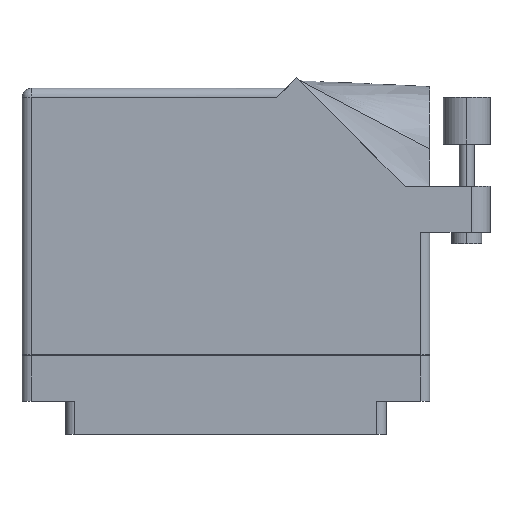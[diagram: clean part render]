
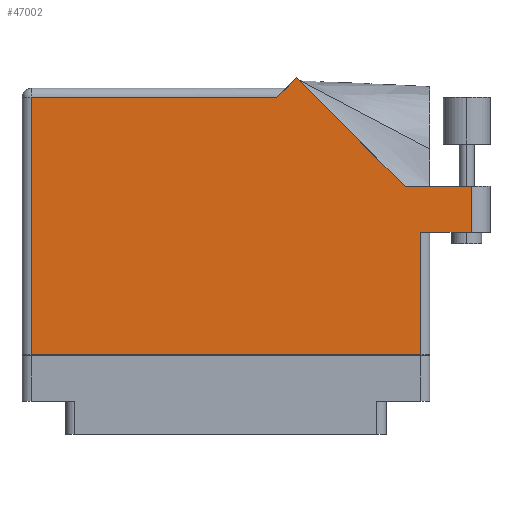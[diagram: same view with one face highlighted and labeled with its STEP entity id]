
A CAD part, front view. The second image highlights one B-rep face of the part: STEP entity #47002.
In plain terms, the highlighted face is planar.
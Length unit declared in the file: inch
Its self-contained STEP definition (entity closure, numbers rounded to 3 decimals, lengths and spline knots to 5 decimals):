
#1333 = VECTOR ( 'NONE', #36020, 39.37008 ) ;
#1382 = CARTESIAN_POINT ( 'NONE',  ( 1.297, 0.715, 0.617 ) ) ;
#3426 = DIRECTION ( 'NONE',  ( -0.707, -0.707, 0. ) ) ;
#3529 = DIRECTION ( 'NONE',  ( -0.707, 0.707, 0. ) ) ;
#4554 = CARTESIAN_POINT ( 'NONE',  ( -1.297, 1.613, 0.617 ) ) ;
#5613 = EDGE_CURVE ( 'NONE', #24596, #61906, #36556, .T. ) ;
#5716 = VECTOR ( 'NONE', #3529, 39.37008 ) ;
#6157 = LINE ( 'NONE', #23024, #23441 ) ;
#6387 = VERTEX_POINT ( 'NONE', #10628 ) ;
#7170 = DIRECTION ( 'NONE',  ( -1., 0., 0. ) ) ;
#8017 = VERTEX_POINT ( 'NONE', #4554 ) ;
#8140 = LINE ( 'NONE', #24655, #5716 ) ;
#8535 = VECTOR ( 'NONE', #12633, 39.37008 ) ;
#9769 = VECTOR ( 'NONE', #3426, 39.37008 ) ;
#10628 = CARTESIAN_POINT ( 'NONE',  ( 0.46971, 1.74571, 0.617 ) ) ;
#12124 = EDGE_CURVE ( 'NONE', #60755, #61768, #32189, .T. ) ;
#12433 = FACE_OUTER_BOUND ( 'NONE', #34349, .T. ) ;
#12633 = DIRECTION ( 'NONE',  ( 0., 1., 0. ) ) ;
#13409 = DIRECTION ( 'NONE',  ( 1., 0., 0. ) ) ;
#15849 = VECTOR ( 'NONE', #68060, 39.37008 ) ;
#16316 = ORIENTED_EDGE ( 'NONE', *, *, #49561, .T. ) ;
#16797 = EDGE_CURVE ( 'NONE', #61906, #49759, #22425, .T. ) ;
#17318 = PLANE ( 'NONE',  #29981 ) ;
#18180 = VECTOR ( 'NONE', #28043, 39.37008 ) ;
#19803 = VECTOR ( 'NONE', #47244, 39.37008 ) ;
#19930 = CARTESIAN_POINT ( 'NONE',  ( -1.297, -0.1, 0.617 ) ) ;
#21676 = EDGE_CURVE ( 'NONE', #6387, #28102, #31180, .T. ) ;
#21844 = CARTESIAN_POINT ( 'NONE',  ( 0.337, 1.613, 0.617 ) ) ;
#22156 = DIRECTION ( 'NONE',  ( -1., 0., 0. ) ) ;
#22425 = LINE ( 'NONE', #41509, #15849 ) ;
#23024 = CARTESIAN_POINT ( 'NONE',  ( 1.359, 0.715, 0.617 ) ) ;
#23441 = VECTOR ( 'NONE', #13409, 39.37008 ) ;
#24087 = CARTESIAN_POINT ( 'NONE',  ( 0.399, 1.675, 0.617 ) ) ;
#24596 = VERTEX_POINT ( 'NONE', #34800 ) ;
#24655 = CARTESIAN_POINT ( 'NONE',  ( 1.19342, 1.022, 0.617 ) ) ;
#27635 = DIRECTION ( 'NONE',  ( 0., 0., -1. ) ) ;
#28043 = DIRECTION ( 'NONE',  ( 0., 1., 0. ) ) ;
#28102 = VERTEX_POINT ( 'NONE', #21844 ) ;
#29981 = AXIS2_PLACEMENT_3D ( 'NONE', #59310, #27635, #22156 ) ;
#31180 = LINE ( 'NONE', #24087, #9769 ) ;
#32120 = LINE ( 'NONE', #52370, #19803 ) ;
#32189 = LINE ( 'NONE', #1382, #18180 ) ;
#33090 = LINE ( 'NONE', #38740, #47942 ) ;
#33174 = CARTESIAN_POINT ( 'NONE',  ( 1.19342, 1.022, 0.617 ) ) ;
#33618 = EDGE_CURVE ( 'NONE', #28102, #8017, #33090, .T. ) ;
#33805 = CARTESIAN_POINT ( 'NONE',  ( 1.634, 1.022, 0.617 ) ) ;
#34349 = EDGE_LOOP ( 'NONE', ( #37007, #57442, #64288, #56884, #44642, #62507, #16316, #34601, #58573 ) ) ;
#34601 = ORIENTED_EDGE ( 'NONE', *, *, #44702, .T. ) ;
#34800 = CARTESIAN_POINT ( 'NONE',  ( 1.634, 0.715, 0.617 ) ) ;
#36020 = DIRECTION ( 'NONE',  ( 0., -1., 0. ) ) ;
#36556 = LINE ( 'NONE', #64951, #8535 ) ;
#37007 = ORIENTED_EDGE ( 'NONE', *, *, #52954, .T. ) ;
#37570 = LINE ( 'NONE', #19930, #1333 ) ;
#38740 = CARTESIAN_POINT ( 'NONE',  ( -1.359, 1.613, 0.617 ) ) ;
#41509 = CARTESIAN_POINT ( 'NONE',  ( 1.759, 1.022, 0.617 ) ) ;
#44642 = ORIENTED_EDGE ( 'NONE', *, *, #21676, .T. ) ;
#44702 = EDGE_CURVE ( 'NONE', #51475, #60755, #32120, .T. ) ;
#47002 = ADVANCED_FACE ( 'NONE', ( #12433 ), #17318, .F. ) ;
#47244 = DIRECTION ( 'NONE',  ( 1., 0., 0. ) ) ;
#47942 = VECTOR ( 'NONE', #7170, 39.37008 ) ;
#49561 = EDGE_CURVE ( 'NONE', #8017, #51475, #37570, .T. ) ;
#49759 = VERTEX_POINT ( 'NONE', #33174 ) ;
#51475 = VERTEX_POINT ( 'NONE', #55315 ) ;
#52370 = CARTESIAN_POINT ( 'NONE',  ( -1.359, -0.1, 0.617 ) ) ;
#52954 = EDGE_CURVE ( 'NONE', #61768, #24596, #6157, .T. ) ;
#54647 = CARTESIAN_POINT ( 'NONE',  ( 1.297, 0.715, 0.617 ) ) ;
#55315 = CARTESIAN_POINT ( 'NONE',  ( -1.297, -0.1, 0.617 ) ) ;
#55379 = CARTESIAN_POINT ( 'NONE',  ( 1.297, -0.1, 0.617 ) ) ;
#56884 = ORIENTED_EDGE ( 'NONE', *, *, #67597, .T. ) ;
#57442 = ORIENTED_EDGE ( 'NONE', *, *, #5613, .T. ) ;
#58573 = ORIENTED_EDGE ( 'NONE', *, *, #12124, .T. ) ;
#59310 = CARTESIAN_POINT ( 'NONE',  ( -1.359, 1.675, 0.617 ) ) ;
#60755 = VERTEX_POINT ( 'NONE', #55379 ) ;
#61768 = VERTEX_POINT ( 'NONE', #54647 ) ;
#61906 = VERTEX_POINT ( 'NONE', #33805 ) ;
#62507 = ORIENTED_EDGE ( 'NONE', *, *, #33618, .T. ) ;
#64288 = ORIENTED_EDGE ( 'NONE', *, *, #16797, .T. ) ;
#64951 = CARTESIAN_POINT ( 'NONE',  ( 1.634, 1.022, 0.617 ) ) ;
#67597 = EDGE_CURVE ( 'NONE', #49759, #6387, #8140, .T. ) ;
#68060 = DIRECTION ( 'NONE',  ( -1., 0., 0. ) ) ;
